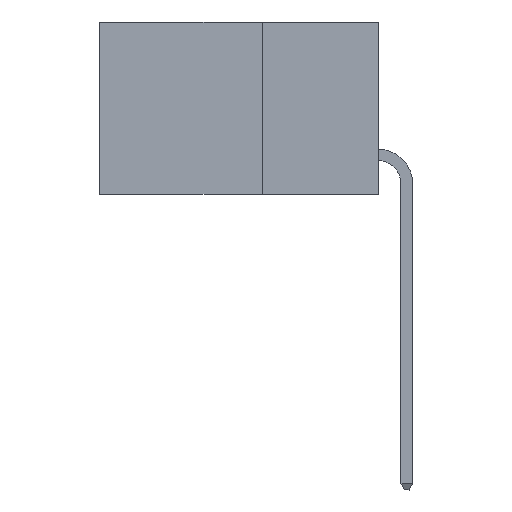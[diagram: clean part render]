
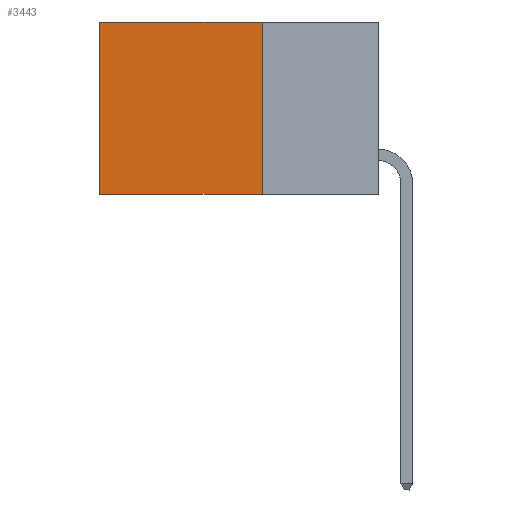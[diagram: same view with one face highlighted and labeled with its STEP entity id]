
A CAD part, left-side view. The second image highlights one B-rep face of the part: STEP entity #3443.
In plain terms, the highlighted planar face has unit normal (-1, 0, 0).
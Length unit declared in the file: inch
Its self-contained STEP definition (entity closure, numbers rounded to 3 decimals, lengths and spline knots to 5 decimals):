
#94 = DIRECTION ( 'NONE',  ( 1., 0., 0. ) ) ;
#291 = ORIENTED_EDGE ( 'NONE', *, *, #4418, .T. ) ;
#674 = EDGE_CURVE ( 'NONE', #3907, #1964, #7719, .T. ) ;
#693 = VERTEX_POINT ( 'NONE', #7294 ) ;
#768 = AXIS2_PLACEMENT_3D ( 'NONE', #7897, #94, #7374 ) ;
#1522 = PLANE ( 'NONE',  #768 ) ;
#1731 = EDGE_CURVE ( 'NONE', #1964, #1833, #10078, .T. ) ;
#1833 = VERTEX_POINT ( 'NONE', #6248 ) ;
#1964 = VERTEX_POINT ( 'NONE', #2222 ) ;
#2222 = CARTESIAN_POINT ( 'NONE',  ( 0.298, 0.25, -0.37 ) ) ;
#2244 = ORIENTED_EDGE ( 'NONE', *, *, #8709, .T. ) ;
#2362 = CARTESIAN_POINT ( 'NONE',  ( 0.298, 0.25, 0. ) ) ;
#2571 = ORIENTED_EDGE ( 'NONE', *, *, #1731, .F. ) ;
#2606 = EDGE_LOOP ( 'NONE', ( #291, #2571, #3559, #2244 ) ) ;
#3136 = CARTESIAN_POINT ( 'NONE',  ( 0.298, 0.25, -0.37 ) ) ;
#3397 = FACE_OUTER_BOUND ( 'NONE', #2606, .T. ) ;
#3443 = ADVANCED_FACE ( 'NONE', ( #3397 ), #1522, .F. ) ;
#3559 = ORIENTED_EDGE ( 'NONE', *, *, #674, .F. ) ;
#3907 = VERTEX_POINT ( 'NONE', #5100 ) ;
#4131 = VECTOR ( 'NONE', #6359, 39.37008 ) ;
#4418 = EDGE_CURVE ( 'NONE', #693, #1833, #6918, .T. ) ;
#4709 = CARTESIAN_POINT ( 'NONE',  ( 0.298, 0.6, 0. ) ) ;
#4941 = VECTOR ( 'NONE', #8045, 39.37008 ) ;
#5100 = CARTESIAN_POINT ( 'NONE',  ( 0.298, 0.25, 0. ) ) ;
#5501 = DIRECTION ( 'NONE',  ( 0., 0., -1. ) ) ;
#6248 = CARTESIAN_POINT ( 'NONE',  ( 0.298, 0.6, -0.37 ) ) ;
#6359 = DIRECTION ( 'NONE',  ( 0., 0., -1. ) ) ;
#6918 = LINE ( 'NONE', #4709, #4131 ) ;
#7294 = CARTESIAN_POINT ( 'NONE',  ( 0.298, 0.6, 0. ) ) ;
#7316 = CARTESIAN_POINT ( 'NONE',  ( 0.298, 0.25, 0. ) ) ;
#7374 = DIRECTION ( 'NONE',  ( 0., 0., -1. ) ) ;
#7446 = VECTOR ( 'NONE', #5501, 39.37008 ) ;
#7719 = LINE ( 'NONE', #2362, #7446 ) ;
#7897 = CARTESIAN_POINT ( 'NONE',  ( 0.298, 0.25, 0. ) ) ;
#8045 = DIRECTION ( 'NONE',  ( 0., 1., 0. ) ) ;
#8542 = VECTOR ( 'NONE', #8927, 39.37008 ) ;
#8709 = EDGE_CURVE ( 'NONE', #3907, #693, #10300, .T. ) ;
#8927 = DIRECTION ( 'NONE',  ( 0., 1., 0. ) ) ;
#10078 = LINE ( 'NONE', #3136, #4941 ) ;
#10300 = LINE ( 'NONE', #7316, #8542 ) ;
